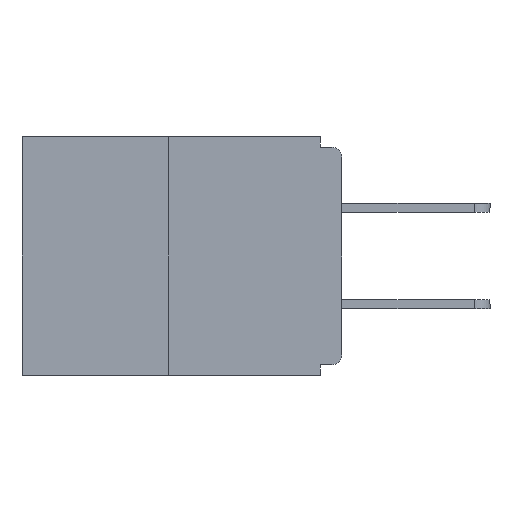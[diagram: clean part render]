
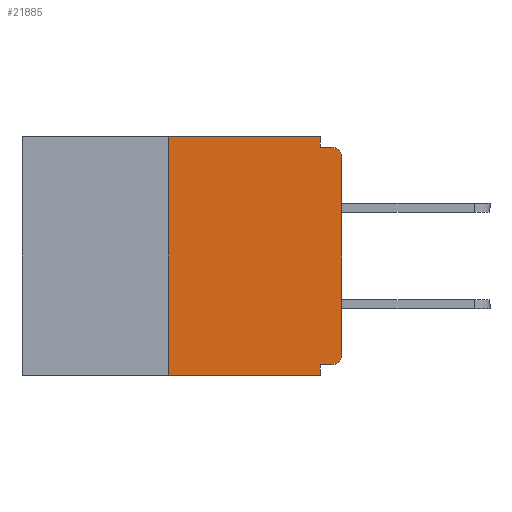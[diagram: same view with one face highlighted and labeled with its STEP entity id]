
A CAD part, left-side view. The second image highlights one B-rep face of the part: STEP entity #21885.
In plain terms, the highlighted planar face has unit normal (-1, 0, 0).
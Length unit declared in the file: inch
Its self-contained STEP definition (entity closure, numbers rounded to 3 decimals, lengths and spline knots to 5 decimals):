
#222 = DIRECTION ( 'NONE',  ( 0., 0., -1. ) ) ;
#291 = DIRECTION ( 'NONE',  ( -1., 0., 0. ) ) ;
#444 = DIRECTION ( 'NONE',  ( 0., -1., 0. ) ) ;
#1002 = DIRECTION ( 'NONE',  ( 0., 0., 1. ) ) ;
#1333 = ORIENTED_EDGE ( 'NONE', *, *, #8415, .F. ) ;
#1432 = CARTESIAN_POINT ( 'NONE',  ( 0., 0.031, -0.343 ) ) ;
#1948 = EDGE_CURVE ( 'NONE', #13140, #6366, #14345, .T. ) ;
#1988 = CARTESIAN_POINT ( 'NONE',  ( 0., 0.46, -0.343 ) ) ;
#2129 = DIRECTION ( 'NONE',  ( 0., -1., 0. ) ) ;
#2144 = LINE ( 'NONE', #1988, #20090 ) ;
#2322 = CARTESIAN_POINT ( 'NONE',  ( 0., 0.015, -0.015 ) ) ;
#3033 = LINE ( 'NONE', #11753, #19077 ) ;
#3174 = DIRECTION ( 'NONE',  ( -1., 0., 0. ) ) ;
#3332 = CARTESIAN_POINT ( 'NONE',  ( 0., 0., 0. ) ) ;
#3850 = VERTEX_POINT ( 'NONE', #22234 ) ;
#4353 = CARTESIAN_POINT ( 'NONE',  ( 0., 0.25, 0. ) ) ;
#4686 = ORIENTED_EDGE ( 'NONE', *, *, #12102, .T. ) ;
#4909 = CARTESIAN_POINT ( 'NONE',  ( 0., 0., -0.328 ) ) ;
#4974 = DIRECTION ( 'NONE',  ( 1., 0., 0. ) ) ;
#5391 = VECTOR ( 'NONE', #12074, 39.37008 ) ;
#6366 = VERTEX_POINT ( 'NONE', #1432 ) ;
#6714 = DIRECTION ( 'NONE',  ( 0., 1., 0. ) ) ;
#6780 = DIRECTION ( 'NONE',  ( 0., 0., -1. ) ) ;
#7273 = LINE ( 'NONE', #21037, #13023 ) ;
#7343 = AXIS2_PLACEMENT_3D ( 'NONE', #14072, #291, #222 ) ;
#7586 = VERTEX_POINT ( 'NONE', #10081 ) ;
#7637 = CARTESIAN_POINT ( 'NONE',  ( 0., 0.031, 0. ) ) ;
#7765 = CIRCLE ( 'NONE', #15952, 0.015 ) ;
#7893 = EDGE_LOOP ( 'NONE', ( #1333, #21070, #16543, #17438, #10511, #4686, #14897, #15736, #9584, #13902 ) ) ;
#8163 = VERTEX_POINT ( 'NONE', #2322 ) ;
#8234 = VERTEX_POINT ( 'NONE', #21021 ) ;
#8415 = EDGE_CURVE ( 'NONE', #7586, #3850, #7273, .T. ) ;
#8869 = LINE ( 'NONE', #4909, #20041 ) ;
#9358 = DIRECTION ( 'NONE',  ( 0., 0., -1. ) ) ;
#9584 = ORIENTED_EDGE ( 'NONE', *, *, #14619, .F. ) ;
#9685 = VERTEX_POINT ( 'NONE', #19532 ) ;
#9726 = CARTESIAN_POINT ( 'NONE',  ( 0., 0.46, 0. ) ) ;
#9936 = EDGE_CURVE ( 'NONE', #17052, #8163, #7765, .T. ) ;
#10081 = CARTESIAN_POINT ( 'NONE',  ( 0., 0.25, 0. ) ) ;
#10433 = CIRCLE ( 'NONE', #7343, 0.015 ) ;
#10499 = VERTEX_POINT ( 'NONE', #14859 ) ;
#10511 = ORIENTED_EDGE ( 'NONE', *, *, #17064, .F. ) ;
#10523 = CARTESIAN_POINT ( 'NONE',  ( 0., 0.015, -0.328 ) ) ;
#10874 = CARTESIAN_POINT ( 'NONE',  ( 0., 0.031, -0.328 ) ) ;
#11035 = CARTESIAN_POINT ( 'NONE',  ( 0., 0.031, -0.343 ) ) ;
#11675 = DIRECTION ( 'NONE',  ( 0., -1., 0. ) ) ;
#11753 = CARTESIAN_POINT ( 'NONE',  ( 0., 0., -0.015 ) ) ;
#11913 = CARTESIAN_POINT ( 'NONE',  ( 0., 0.015, -0.03 ) ) ;
#12074 = DIRECTION ( 'NONE',  ( 0., 0., 1. ) ) ;
#12102 = EDGE_CURVE ( 'NONE', #16291, #10499, #10433, .T. ) ;
#12239 = LINE ( 'NONE', #3332, #5391 ) ;
#12282 = LINE ( 'NONE', #7637, #15531 ) ;
#13023 = VECTOR ( 'NONE', #444, 39.37008 ) ;
#13140 = VERTEX_POINT ( 'NONE', #10874 ) ;
#13251 = EDGE_CURVE ( 'NONE', #9685, #7586, #21010, .T. ) ;
#13902 = ORIENTED_EDGE ( 'NONE', *, *, #15049, .F. ) ;
#14072 = CARTESIAN_POINT ( 'NONE',  ( 0., 0.015, -0.313 ) ) ;
#14345 = LINE ( 'NONE', #11035, #21097 ) ;
#14619 = EDGE_CURVE ( 'NONE', #8234, #8163, #3033, .T. ) ;
#14859 = CARTESIAN_POINT ( 'NONE',  ( 0., 0., -0.313 ) ) ;
#14897 = ORIENTED_EDGE ( 'NONE', *, *, #15962, .T. ) ;
#15049 = EDGE_CURVE ( 'NONE', #3850, #8234, #12282, .T. ) ;
#15531 = VECTOR ( 'NONE', #9358, 39.37008 ) ;
#15736 = ORIENTED_EDGE ( 'NONE', *, *, #9936, .T. ) ;
#15952 = AXIS2_PLACEMENT_3D ( 'NONE', #11913, #3174, #18510 ) ;
#15962 = EDGE_CURVE ( 'NONE', #10499, #17052, #12239, .T. ) ;
#16291 = VERTEX_POINT ( 'NONE', #10523 ) ;
#16450 = DIRECTION ( 'NONE',  ( 0., 0., -1. ) ) ;
#16543 = ORIENTED_EDGE ( 'NONE', *, *, #21634, .T. ) ;
#16853 = AXIS2_PLACEMENT_3D ( 'NONE', #9726, #4974, #6780 ) ;
#17052 = VERTEX_POINT ( 'NONE', #18894 ) ;
#17064 = EDGE_CURVE ( 'NONE', #16291, #13140, #8869, .T. ) ;
#17438 = ORIENTED_EDGE ( 'NONE', *, *, #1948, .F. ) ;
#18510 = DIRECTION ( 'NONE',  ( 0., 0., -1. ) ) ;
#18894 = CARTESIAN_POINT ( 'NONE',  ( 0., 0., -0.03 ) ) ;
#19077 = VECTOR ( 'NONE', #11675, 39.37008 ) ;
#19532 = CARTESIAN_POINT ( 'NONE',  ( 0., 0.25, -0.343 ) ) ;
#20041 = VECTOR ( 'NONE', #6714, 39.37008 ) ;
#20090 = VECTOR ( 'NONE', #2129, 39.37008 ) ;
#20200 = PLANE ( 'NONE',  #16853 ) ;
#21010 = LINE ( 'NONE', #4353, #21806 ) ;
#21021 = CARTESIAN_POINT ( 'NONE',  ( 0., 0.031, -0.015 ) ) ;
#21037 = CARTESIAN_POINT ( 'NONE',  ( 0., 0.46, 0. ) ) ;
#21070 = ORIENTED_EDGE ( 'NONE', *, *, #13251, .F. ) ;
#21097 = VECTOR ( 'NONE', #16450, 39.37008 ) ;
#21634 = EDGE_CURVE ( 'NONE', #9685, #6366, #2144, .T. ) ;
#21806 = VECTOR ( 'NONE', #1002, 39.37008 ) ;
#21885 = ADVANCED_FACE ( 'NONE', ( #22126 ), #20200, .F. ) ;
#22126 = FACE_OUTER_BOUND ( 'NONE', #7893, .T. ) ;
#22234 = CARTESIAN_POINT ( 'NONE',  ( 0., 0.031, 0. ) ) ;
